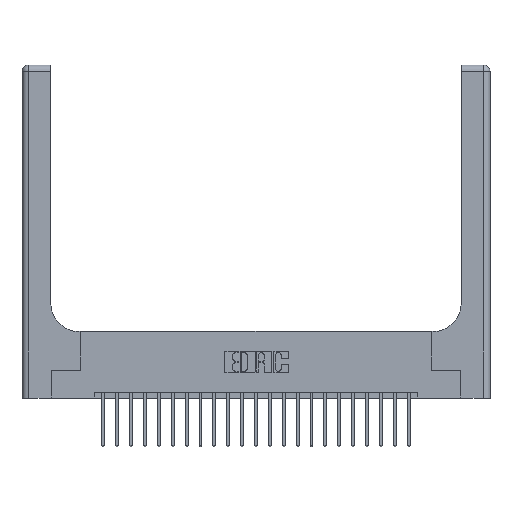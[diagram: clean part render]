
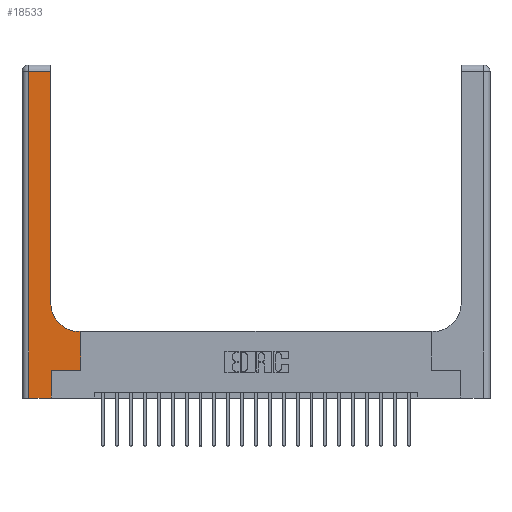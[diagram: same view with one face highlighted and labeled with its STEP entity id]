
A CAD part, top view. The second image highlights one B-rep face of the part: STEP entity #18533.
In plain terms, the highlighted planar face has unit normal (0, 0, 1).
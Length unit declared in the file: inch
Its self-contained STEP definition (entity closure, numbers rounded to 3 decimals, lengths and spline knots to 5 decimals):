
#273 = EDGE_CURVE ( 'NONE', #17939, #12359, #20548, .T. ) ;
#848 = CARTESIAN_POINT ( 'NONE',  ( 0.528, 0.6, 0.37 ) ) ;
#2146 = LINE ( 'NONE', #12064, #20299 ) ;
#2445 = EDGE_CURVE ( 'NONE', #18427, #12571, #15540, .T. ) ;
#2569 = CARTESIAN_POINT ( 'NONE',  ( 0.06, 2.94, 0.37 ) ) ;
#2870 = LINE ( 'NONE', #2923, #13901 ) ;
#2923 = CARTESIAN_POINT ( 'NONE',  ( 0.06, 3., 0.37 ) ) ;
#2959 = VERTEX_POINT ( 'NONE', #848 ) ;
#3159 = DIRECTION ( 'NONE',  ( 1., 0., 0. ) ) ;
#3456 = CARTESIAN_POINT ( 'NONE',  ( 0.265, 0.25, 0.37 ) ) ;
#4205 = ORIENTED_EDGE ( 'NONE', *, *, #18825, .T. ) ;
#4313 = LINE ( 'NONE', #5970, #7870 ) ;
#5274 = EDGE_CURVE ( 'NONE', #12571, #18301, #2870, .T. ) ;
#5970 = CARTESIAN_POINT ( 'NONE',  ( 0.528, 0.25, 0.37 ) ) ;
#6374 = LINE ( 'NONE', #19087, #14082 ) ;
#6663 = AXIS2_PLACEMENT_3D ( 'NONE', #18820, #15465, #16859 ) ;
#6908 = DIRECTION ( 'NONE',  ( 0., 1., 0. ) ) ;
#6993 = VECTOR ( 'NONE', #13914, 39.37008 ) ;
#7461 = CARTESIAN_POINT ( 'NONE',  ( 0.06, 0., 0.37 ) ) ;
#7870 = VECTOR ( 'NONE', #16432, 39.37008 ) ;
#7876 = CARTESIAN_POINT ( 'NONE',  ( 0.265, 0.25, 0.37 ) ) ;
#8522 = EDGE_CURVE ( 'NONE', #17630, #8786, #19766, .T. ) ;
#8620 = AXIS2_PLACEMENT_3D ( 'NONE', #15832, #21064, #12193 ) ;
#8786 = VERTEX_POINT ( 'NONE', #3456 ) ;
#9157 = EDGE_LOOP ( 'NONE', ( #13559, #13635, #16467, #11267, #17420, #10964, #12530, #4205, #9753 ) ) ;
#9753 = ORIENTED_EDGE ( 'NONE', *, *, #273, .T. ) ;
#10876 = DIRECTION ( 'NONE',  ( -1., 0., 0. ) ) ;
#10964 = ORIENTED_EDGE ( 'NONE', *, *, #17368, .T. ) ;
#11267 = ORIENTED_EDGE ( 'NONE', *, *, #16093, .T. ) ;
#11903 = PLANE ( 'NONE',  #6663 ) ;
#12064 = CARTESIAN_POINT ( 'NONE',  ( 0., 0., 0.37 ) ) ;
#12126 = CARTESIAN_POINT ( 'NONE',  ( 0.265, 0., 0.37 ) ) ;
#12193 = DIRECTION ( 'NONE',  ( 1., 0., 0. ) ) ;
#12359 = VERTEX_POINT ( 'NONE', #19428 ) ;
#12530 = ORIENTED_EDGE ( 'NONE', *, *, #21731, .T. ) ;
#12571 = VERTEX_POINT ( 'NONE', #2569 ) ;
#13047 = DIRECTION ( 'NONE',  ( 1., 0., 0. ) ) ;
#13053 = CARTESIAN_POINT ( 'NONE',  ( 0.26, 2.94, 0.37 ) ) ;
#13209 = CARTESIAN_POINT ( 'NONE',  ( 0.528, 0.25, 0.37 ) ) ;
#13408 = LINE ( 'NONE', #7876, #18440 ) ;
#13553 = DIRECTION ( 'NONE',  ( 0., -1., 0. ) ) ;
#13559 = ORIENTED_EDGE ( 'NONE', *, *, #19733, .T. ) ;
#13635 = ORIENTED_EDGE ( 'NONE', *, *, #2445, .T. ) ;
#13718 = DIRECTION ( 'NONE',  ( 0., 1., 0. ) ) ;
#13901 = VECTOR ( 'NONE', #13553, 39.37008 ) ;
#13914 = DIRECTION ( 'NONE',  ( -1., 0., 0. ) ) ;
#14082 = VECTOR ( 'NONE', #13718, 39.37008 ) ;
#15112 = VECTOR ( 'NONE', #6908, 39.37008 ) ;
#15226 = VECTOR ( 'NONE', #10876, 39.37008 ) ;
#15465 = DIRECTION ( 'NONE',  ( 0., 0., -1. ) ) ;
#15540 = LINE ( 'NONE', #22603, #6993 ) ;
#15832 = CARTESIAN_POINT ( 'NONE',  ( 0.51, 0.85, 0.37 ) ) ;
#16052 = CARTESIAN_POINT ( 'NONE',  ( 0.51, 0.6, 0.37 ) ) ;
#16073 = FACE_OUTER_BOUND ( 'NONE', #9157, .T. ) ;
#16093 = EDGE_CURVE ( 'NONE', #18301, #17630, #2146, .T. ) ;
#16432 = DIRECTION ( 'NONE',  ( 0., 1., 0. ) ) ;
#16467 = ORIENTED_EDGE ( 'NONE', *, *, #5274, .T. ) ;
#16859 = DIRECTION ( 'NONE',  ( -1., 0., 0. ) ) ;
#17368 = EDGE_CURVE ( 'NONE', #8786, #21405, #13408, .T. ) ;
#17420 = ORIENTED_EDGE ( 'NONE', *, *, #8522, .T. ) ;
#17630 = VERTEX_POINT ( 'NONE', #12126 ) ;
#17749 = CARTESIAN_POINT ( 'NONE',  ( 0.26, 0.6, 0.37 ) ) ;
#17939 = VERTEX_POINT ( 'NONE', #16052 ) ;
#18301 = VERTEX_POINT ( 'NONE', #7461 ) ;
#18427 = VERTEX_POINT ( 'NONE', #13053 ) ;
#18440 = VECTOR ( 'NONE', #13047, 39.37008 ) ;
#18533 = ADVANCED_FACE ( 'NONE', ( #16073 ), #11903, .F. ) ;
#18820 = CARTESIAN_POINT ( 'NONE',  ( 0., 3., 0.37 ) ) ;
#18825 = EDGE_CURVE ( 'NONE', #2959, #17939, #19881, .T. ) ;
#19087 = CARTESIAN_POINT ( 'NONE',  ( 0.26, 3., 0.37 ) ) ;
#19428 = CARTESIAN_POINT ( 'NONE',  ( 0.26, 0.85, 0.37 ) ) ;
#19733 = EDGE_CURVE ( 'NONE', #12359, #18427, #6374, .T. ) ;
#19766 = LINE ( 'NONE', #21140, #15112 ) ;
#19881 = LINE ( 'NONE', #17749, #15226 ) ;
#20299 = VECTOR ( 'NONE', #3159, 39.37008 ) ;
#20548 = CIRCLE ( 'NONE', #8620, 0.25 ) ;
#21064 = DIRECTION ( 'NONE',  ( 0., 0., -1. ) ) ;
#21140 = CARTESIAN_POINT ( 'NONE',  ( 0.265, 0., 0.37 ) ) ;
#21405 = VERTEX_POINT ( 'NONE', #13209 ) ;
#21731 = EDGE_CURVE ( 'NONE', #21405, #2959, #4313, .T. ) ;
#22603 = CARTESIAN_POINT ( 'NONE',  ( 0., 2.94, 0.37 ) ) ;
